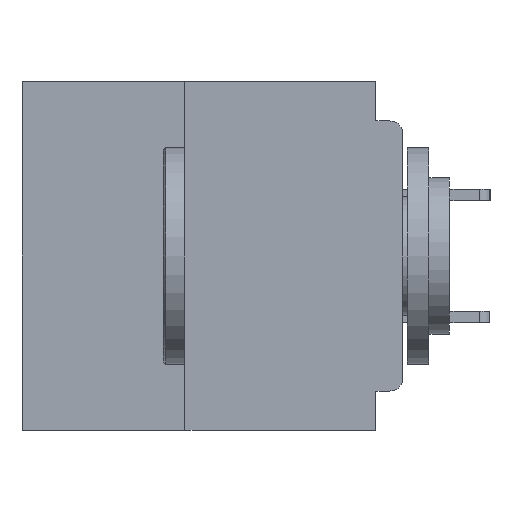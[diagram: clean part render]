
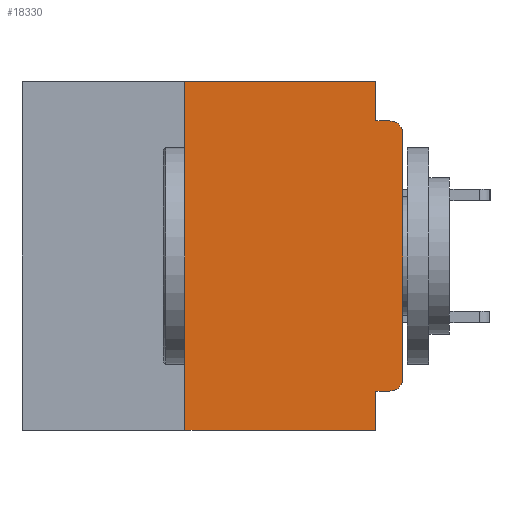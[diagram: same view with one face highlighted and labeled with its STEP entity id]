
A CAD part, left-side view. The second image highlights one B-rep face of the part: STEP entity #18330.
In plain terms, the highlighted planar face has unit normal (-1, 0, 0).
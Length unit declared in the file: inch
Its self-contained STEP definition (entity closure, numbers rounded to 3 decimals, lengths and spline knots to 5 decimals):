
#1121 = AXIS2_PLACEMENT_3D ( 'NONE', #40240, #18773, #43809 ) ;
#2203 = EDGE_CURVE ( 'NONE', #39948, #29967, #36474, .T. ) ;
#4080 = ORIENTED_EDGE ( 'NONE', *, *, #12577, .F. ) ;
#4820 = EDGE_CURVE ( 'NONE', #20699, #6188, #11232, .T. ) ;
#4985 = DIRECTION ( 'NONE',  ( 1., 0., 0. ) ) ;
#5533 = VECTOR ( 'NONE', #43841, 39.37008 ) ;
#6188 = VERTEX_POINT ( 'NONE', #33473 ) ;
#6311 = CARTESIAN_POINT ( 'NONE',  ( 0., 0., -0.06 ) ) ;
#6466 = ORIENTED_EDGE ( 'NONE', *, *, #12586, .T. ) ;
#7495 = CARTESIAN_POINT ( 'NONE',  ( 0., 0.25, 0. ) ) ;
#8023 = CARTESIAN_POINT ( 'NONE',  ( 0., 0., 0. ) ) ;
#8123 = CARTESIAN_POINT ( 'NONE',  ( 0., 0.25, -0.4 ) ) ;
#8187 = CARTESIAN_POINT ( 'NONE',  ( 0., 0.25, -0.4 ) ) ;
#8734 = CARTESIAN_POINT ( 'NONE',  ( 0., 0.015, -0.34 ) ) ;
#8920 = LINE ( 'NONE', #13823, #26911 ) ;
#9344 = ORIENTED_EDGE ( 'NONE', *, *, #18956, .T. ) ;
#10108 = ORIENTED_EDGE ( 'NONE', *, *, #30041, .F. ) ;
#10622 = EDGE_CURVE ( 'NONE', #28631, #29967, #13955, .T. ) ;
#10731 = CARTESIAN_POINT ( 'NONE',  ( 0., 0.031, -0.4 ) ) ;
#10778 = CARTESIAN_POINT ( 'NONE',  ( 0., 0.031, -0.355 ) ) ;
#10804 = DIRECTION ( 'NONE',  ( 0., -1., 0. ) ) ;
#10869 = LINE ( 'NONE', #8023, #20439 ) ;
#11232 = LINE ( 'NONE', #20697, #30267 ) ;
#11488 = EDGE_CURVE ( 'NONE', #32604, #20699, #25623, .T. ) ;
#11737 = ORIENTED_EDGE ( 'NONE', *, *, #35703, .F. ) ;
#11857 = DIRECTION ( 'NONE',  ( 0., 0., 1. ) ) ;
#12404 = DIRECTION ( 'NONE',  ( 0., 0., -1. ) ) ;
#12577 = EDGE_CURVE ( 'NONE', #31804, #43260, #17697, .T. ) ;
#12586 = EDGE_CURVE ( 'NONE', #32604, #44822, #35621, .T. ) ;
#13409 = AXIS2_PLACEMENT_3D ( 'NONE', #8734, #33817, #12404 ) ;
#13501 = CARTESIAN_POINT ( 'NONE',  ( 0., 0.031, -0.045 ) ) ;
#13823 = CARTESIAN_POINT ( 'NONE',  ( 0., 0.031, 0. ) ) ;
#13955 = CIRCLE ( 'NONE', #1121, 0.015 ) ;
#15161 = LINE ( 'NONE', #18805, #5533 ) ;
#15182 = AXIS2_PLACEMENT_3D ( 'NONE', #19358, #4985, #30128 ) ;
#15632 = VERTEX_POINT ( 'NONE', #39809 ) ;
#15737 = PLANE ( 'NONE',  #15182 ) ;
#16868 = EDGE_LOOP ( 'NONE', ( #44416, #19014, #34760, #11737, #26082, #33502, #6466, #10108, #4080, #9344 ) ) ;
#17428 = DIRECTION ( 'NONE',  ( 0., 0., -1. ) ) ;
#17697 = LINE ( 'NONE', #39507, #27194 ) ;
#18036 = CARTESIAN_POINT ( 'NONE',  ( 0., 0.437, -0.4 ) ) ;
#18330 = ADVANCED_FACE ( 'NONE', ( #39202 ), #15737, .F. ) ;
#18773 = DIRECTION ( 'NONE',  ( -1., 0., 0. ) ) ;
#18805 = CARTESIAN_POINT ( 'NONE',  ( 0., 0.031, -0.4 ) ) ;
#18956 = EDGE_CURVE ( 'NONE', #31804, #15632, #39712, .T. ) ;
#19014 = ORIENTED_EDGE ( 'NONE', *, *, #10622, .T. ) ;
#19358 = CARTESIAN_POINT ( 'NONE',  ( 0., 0.437, 0. ) ) ;
#19874 = DIRECTION ( 'NONE',  ( 0., -1., 0. ) ) ;
#20439 = VECTOR ( 'NONE', #25925, 39.37008 ) ;
#20697 = CARTESIAN_POINT ( 'NONE',  ( 0., 0.437, 0. ) ) ;
#20699 = VERTEX_POINT ( 'NONE', #7495 ) ;
#25623 = LINE ( 'NONE', #8187, #43553 ) ;
#25925 = DIRECTION ( 'NONE',  ( 0., 0., 1. ) ) ;
#26082 = ORIENTED_EDGE ( 'NONE', *, *, #4820, .F. ) ;
#26911 = VECTOR ( 'NONE', #17428, 39.37008 ) ;
#26919 = VECTOR ( 'NONE', #43434, 39.37008 ) ;
#27194 = VECTOR ( 'NONE', #43062, 39.37008 ) ;
#28116 = EDGE_CURVE ( 'NONE', #15632, #28631, #10869, .T. ) ;
#28631 = VERTEX_POINT ( 'NONE', #6311 ) ;
#29967 = VERTEX_POINT ( 'NONE', #39672 ) ;
#30041 = EDGE_CURVE ( 'NONE', #43260, #44822, #15161, .T. ) ;
#30128 = DIRECTION ( 'NONE',  ( 0., 0., -1. ) ) ;
#30267 = VECTOR ( 'NONE', #19874, 39.37008 ) ;
#31804 = VERTEX_POINT ( 'NONE', #42389 ) ;
#32604 = VERTEX_POINT ( 'NONE', #8123 ) ;
#33473 = CARTESIAN_POINT ( 'NONE',  ( 0., 0.031, 0. ) ) ;
#33502 = ORIENTED_EDGE ( 'NONE', *, *, #11488, .F. ) ;
#33817 = DIRECTION ( 'NONE',  ( -1., 0., 0. ) ) ;
#34461 = VECTOR ( 'NONE', #10804, 39.37008 ) ;
#34760 = ORIENTED_EDGE ( 'NONE', *, *, #2203, .F. ) ;
#35621 = LINE ( 'NONE', #18036, #34461 ) ;
#35703 = EDGE_CURVE ( 'NONE', #6188, #39948, #8920, .T. ) ;
#36474 = LINE ( 'NONE', #45876, #26919 ) ;
#39202 = FACE_OUTER_BOUND ( 'NONE', #16868, .T. ) ;
#39507 = CARTESIAN_POINT ( 'NONE',  ( 0., 0., -0.355 ) ) ;
#39672 = CARTESIAN_POINT ( 'NONE',  ( 0., 0.015, -0.045 ) ) ;
#39712 = CIRCLE ( 'NONE', #13409, 0.015 ) ;
#39809 = CARTESIAN_POINT ( 'NONE',  ( 0., 0., -0.34 ) ) ;
#39948 = VERTEX_POINT ( 'NONE', #13501 ) ;
#40240 = CARTESIAN_POINT ( 'NONE',  ( 0., 0.015, -0.06 ) ) ;
#42389 = CARTESIAN_POINT ( 'NONE',  ( 0., 0.015, -0.355 ) ) ;
#43062 = DIRECTION ( 'NONE',  ( 0., 1., 0. ) ) ;
#43260 = VERTEX_POINT ( 'NONE', #10778 ) ;
#43434 = DIRECTION ( 'NONE',  ( 0., -1., 0. ) ) ;
#43553 = VECTOR ( 'NONE', #11857, 39.37008 ) ;
#43809 = DIRECTION ( 'NONE',  ( 0., 0., -1. ) ) ;
#43841 = DIRECTION ( 'NONE',  ( 0., 0., -1. ) ) ;
#44416 = ORIENTED_EDGE ( 'NONE', *, *, #28116, .T. ) ;
#44822 = VERTEX_POINT ( 'NONE', #10731 ) ;
#45876 = CARTESIAN_POINT ( 'NONE',  ( 0., 0., -0.045 ) ) ;
